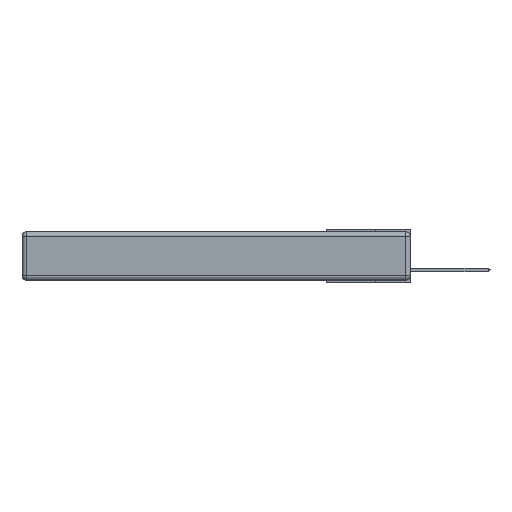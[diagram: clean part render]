
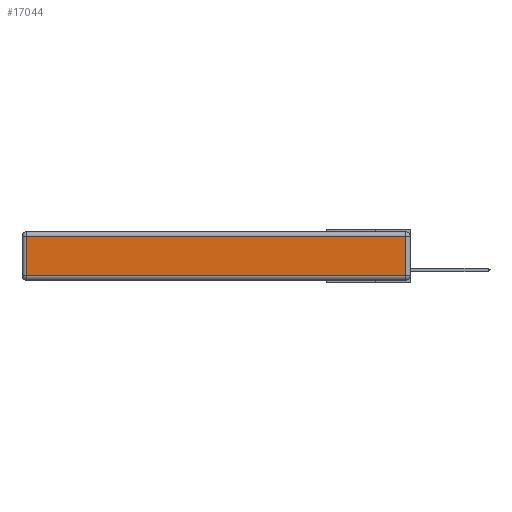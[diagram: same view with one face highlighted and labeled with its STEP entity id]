
A CAD part, left-side view. The second image highlights one B-rep face of the part: STEP entity #17044.
In plain terms, the highlighted planar face has unit normal (-1, 0, 0).
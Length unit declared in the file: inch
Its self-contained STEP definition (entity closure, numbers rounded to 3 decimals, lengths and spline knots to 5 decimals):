
#118 = CARTESIAN_POINT ( 'NONE',  ( 0., 0.03, -0.313 ) ) ;
#206 = CARTESIAN_POINT ( 'NONE',  ( 0., 2.72, -0.343 ) ) ;
#211 = EDGE_LOOP ( 'NONE', ( #22473, #8118, #10313, #3882 ) ) ;
#1490 = CARTESIAN_POINT ( 'NONE',  ( 0., 0., -0.343 ) ) ;
#1968 = EDGE_CURVE ( 'NONE', #24709, #9746, #20758, .T. ) ;
#2838 = CARTESIAN_POINT ( 'NONE',  ( 0., 2.72, -0.03 ) ) ;
#3882 = ORIENTED_EDGE ( 'NONE', *, *, #1968, .T. ) ;
#4827 = DIRECTION ( 'NONE',  ( 0., 1., 0. ) ) ;
#4897 = VERTEX_POINT ( 'NONE', #118 ) ;
#5414 = VERTEX_POINT ( 'NONE', #22107 ) ;
#6393 = EDGE_CURVE ( 'NONE', #9746, #4897, #22038, .T. ) ;
#6949 = EDGE_CURVE ( 'NONE', #4897, #5414, #16936, .T. ) ;
#7276 = DIRECTION ( 'NONE',  ( 0., 0., 1. ) ) ;
#7504 = CARTESIAN_POINT ( 'NONE',  ( 0., 2.72, -0.313 ) ) ;
#7919 = VECTOR ( 'NONE', #13620, 39.37008 ) ;
#8055 = DIRECTION ( 'NONE',  ( 0., 0., 1. ) ) ;
#8118 = ORIENTED_EDGE ( 'NONE', *, *, #6949, .T. ) ;
#9746 = VERTEX_POINT ( 'NONE', #7504 ) ;
#10313 = ORIENTED_EDGE ( 'NONE', *, *, #16259, .T. ) ;
#13620 = DIRECTION ( 'NONE',  ( 0., 0., -1. ) ) ;
#16259 = EDGE_CURVE ( 'NONE', #5414, #24709, #20311, .T. ) ;
#16657 = CARTESIAN_POINT ( 'NONE',  ( 0., 0., -0.313 ) ) ;
#16936 = LINE ( 'NONE', #23265, #18148 ) ;
#17044 = ADVANCED_FACE ( 'NONE', ( #21470 ), #24399, .T. ) ;
#18148 = VECTOR ( 'NONE', #8055, 39.37008 ) ;
#18725 = DIRECTION ( 'NONE',  ( -1., 0., 0. ) ) ;
#18915 = AXIS2_PLACEMENT_3D ( 'NONE', #1490, #18725, #7276 ) ;
#20311 = LINE ( 'NONE', #21776, #23889 ) ;
#20412 = DIRECTION ( 'NONE',  ( 0., -1., 0. ) ) ;
#20758 = LINE ( 'NONE', #206, #7919 ) ;
#21470 = FACE_OUTER_BOUND ( 'NONE', #211, .T. ) ;
#21776 = CARTESIAN_POINT ( 'NONE',  ( 0., 2.75, -0.03 ) ) ;
#22038 = LINE ( 'NONE', #16657, #23213 ) ;
#22107 = CARTESIAN_POINT ( 'NONE',  ( 0., 0.03, -0.03 ) ) ;
#22473 = ORIENTED_EDGE ( 'NONE', *, *, #6393, .T. ) ;
#23213 = VECTOR ( 'NONE', #20412, 39.37008 ) ;
#23265 = CARTESIAN_POINT ( 'NONE',  ( 0., 0.03, -0.343 ) ) ;
#23889 = VECTOR ( 'NONE', #4827, 39.37008 ) ;
#24399 = PLANE ( 'NONE',  #18915 ) ;
#24709 = VERTEX_POINT ( 'NONE', #2838 ) ;
